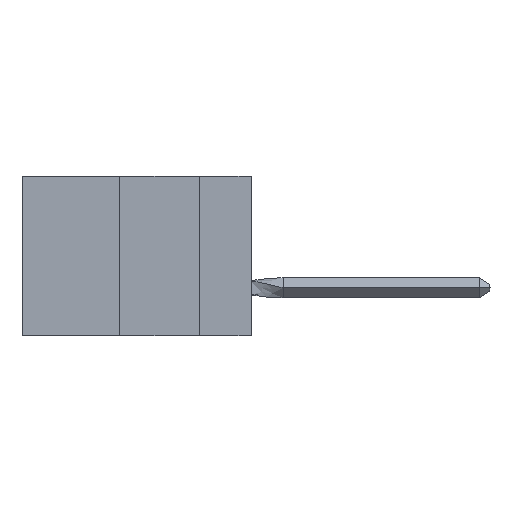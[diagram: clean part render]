
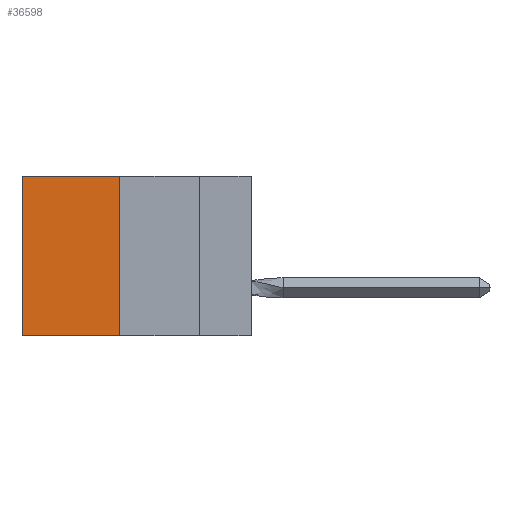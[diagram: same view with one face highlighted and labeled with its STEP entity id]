
A CAD part, left-side view. The second image highlights one B-rep face of the part: STEP entity #36598.
In plain terms, the highlighted planar face has unit normal (-1, 0, 0).
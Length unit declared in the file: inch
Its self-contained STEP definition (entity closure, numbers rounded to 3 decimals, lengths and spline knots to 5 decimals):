
#4960 = CARTESIAN_POINT ( 'NONE',  ( 0.305, 0.72, -0.5 ) ) ;
#5873 = EDGE_CURVE ( 'NONE', #36715, #31029, #22367, .T. ) ;
#7180 = LINE ( 'NONE', #38883, #18459 ) ;
#8552 = LINE ( 'NONE', #24740, #32503 ) ;
#9064 = DIRECTION ( 'NONE',  ( 0., 0., -1. ) ) ;
#10989 = CARTESIAN_POINT ( 'NONE',  ( 0.305, 0.413, -0.5 ) ) ;
#11399 = DIRECTION ( 'NONE',  ( 0., 1., 0. ) ) ;
#12534 = VERTEX_POINT ( 'NONE', #27740 ) ;
#12631 = AXIS2_PLACEMENT_3D ( 'NONE', #21996, #38387, #19545 ) ;
#14564 = FACE_OUTER_BOUND ( 'NONE', #33692, .T. ) ;
#14951 = ORIENTED_EDGE ( 'NONE', *, *, #5873, .F. ) ;
#16073 = VECTOR ( 'NONE', #11399, 39.37008 ) ;
#17158 = ORIENTED_EDGE ( 'NONE', *, *, #31959, .T. ) ;
#18459 = VECTOR ( 'NONE', #19927, 39.37008 ) ;
#18659 = CARTESIAN_POINT ( 'NONE',  ( 0.305, 0.413, 0. ) ) ;
#19545 = DIRECTION ( 'NONE',  ( 0., 0., -1. ) ) ;
#19927 = DIRECTION ( 'NONE',  ( 0., 0., -1. ) ) ;
#21555 = DIRECTION ( 'NONE',  ( 0., 1., 0. ) ) ;
#21996 = CARTESIAN_POINT ( 'NONE',  ( 0.305, 0.413, -0.5 ) ) ;
#22367 = LINE ( 'NONE', #10989, #16073 ) ;
#24709 = ORIENTED_EDGE ( 'NONE', *, *, #37937, .T. ) ;
#24740 = CARTESIAN_POINT ( 'NONE',  ( 0.305, 0.413, -0.5 ) ) ;
#25712 = VECTOR ( 'NONE', #21555, 39.37008 ) ;
#27740 = CARTESIAN_POINT ( 'NONE',  ( 0.305, 0.72, 0. ) ) ;
#28758 = ORIENTED_EDGE ( 'NONE', *, *, #32689, .F. ) ;
#31029 = VERTEX_POINT ( 'NONE', #4960 ) ;
#31079 = CARTESIAN_POINT ( 'NONE',  ( 0.305, 0.413, 0. ) ) ;
#31959 = EDGE_CURVE ( 'NONE', #35985, #12534, #32072, .T. ) ;
#32072 = LINE ( 'NONE', #31079, #25712 ) ;
#32503 = VECTOR ( 'NONE', #9064, 39.37008 ) ;
#32689 = EDGE_CURVE ( 'NONE', #35985, #36715, #8552, .T. ) ;
#33692 = EDGE_LOOP ( 'NONE', ( #24709, #14951, #28758, #17158 ) ) ;
#35985 = VERTEX_POINT ( 'NONE', #18659 ) ;
#36440 = CARTESIAN_POINT ( 'NONE',  ( 0.305, 0.413, -0.5 ) ) ;
#36598 = ADVANCED_FACE ( 'NONE', ( #14564 ), #37551, .F. ) ;
#36715 = VERTEX_POINT ( 'NONE', #36440 ) ;
#37551 = PLANE ( 'NONE',  #12631 ) ;
#37937 = EDGE_CURVE ( 'NONE', #12534, #31029, #7180, .T. ) ;
#38387 = DIRECTION ( 'NONE',  ( 1., 0., 0. ) ) ;
#38883 = CARTESIAN_POINT ( 'NONE',  ( 0.305, 0.72, -0.5 ) ) ;
